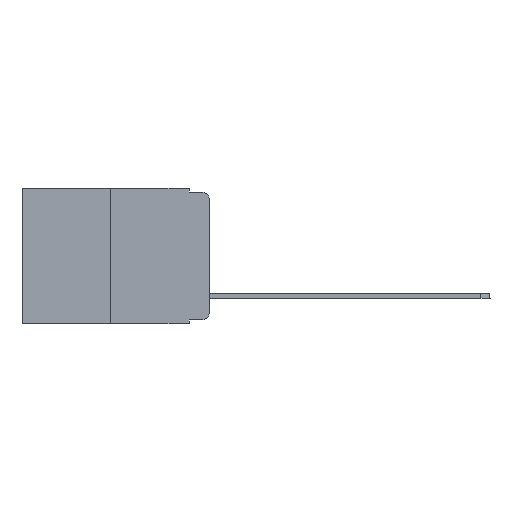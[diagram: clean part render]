
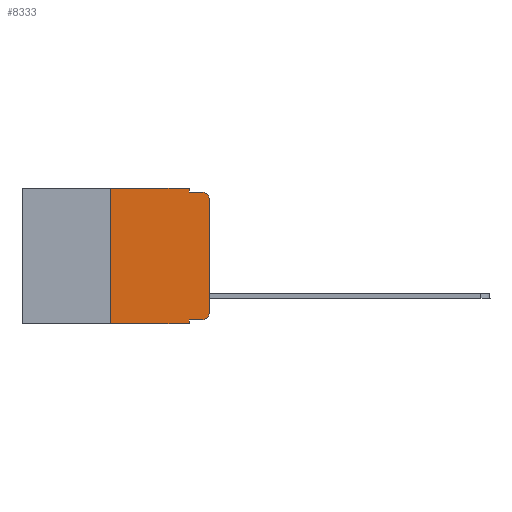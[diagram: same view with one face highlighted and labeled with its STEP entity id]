
A CAD part, left-side view. The second image highlights one B-rep face of the part: STEP entity #8333.
In plain terms, the highlighted planar face has unit normal (-1, 0, 0).
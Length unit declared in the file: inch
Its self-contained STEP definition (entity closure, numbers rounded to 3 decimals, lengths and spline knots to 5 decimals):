
#16 = VERTEX_POINT ( 'NONE', #17097 ) ;
#39 = VECTOR ( 'NONE', #5047, 39.37008 ) ;
#116 = CARTESIAN_POINT ( 'NONE',  ( 0., 0.051, 0. ) ) ;
#132 = EDGE_CURVE ( 'NONE', #12081, #515, #3563, .T. ) ;
#515 = VERTEX_POINT ( 'NONE', #19329 ) ;
#526 = CARTESIAN_POINT ( 'NONE',  ( 0., 0., -0.03 ) ) ;
#568 = EDGE_CURVE ( 'NONE', #9668, #515, #5757, .T. ) ;
#625 = ORIENTED_EDGE ( 'NONE', *, *, #12932, .F. ) ;
#695 = CARTESIAN_POINT ( 'NONE',  ( 0., 0.051, -0.333 ) ) ;
#789 = ORIENTED_EDGE ( 'NONE', *, *, #18024, .T. ) ;
#1224 = CARTESIAN_POINT ( 'NONE',  ( 0., 0.02, -0.333 ) ) ;
#1557 = ORIENTED_EDGE ( 'NONE', *, *, #5802, .T. ) ;
#1624 = ORIENTED_EDGE ( 'NONE', *, *, #2124, .F. ) ;
#1813 = CARTESIAN_POINT ( 'NONE',  ( 0., 0.051, -0.01 ) ) ;
#2092 = ORIENTED_EDGE ( 'NONE', *, *, #11781, .T. ) ;
#2124 = EDGE_CURVE ( 'NONE', #16144, #4587, #16468, .T. ) ;
#2395 = VERTEX_POINT ( 'NONE', #3873 ) ;
#2454 = CARTESIAN_POINT ( 'NONE',  ( 0., 0.473, -0.343 ) ) ;
#2732 = CIRCLE ( 'NONE', #10613, 0.02 ) ;
#2763 = CARTESIAN_POINT ( 'NONE',  ( 0., 0.051, 0. ) ) ;
#2802 = DIRECTION ( 'NONE',  ( -1., 0., 0. ) ) ;
#2873 = DIRECTION ( 'NONE',  ( 1., 0., 0. ) ) ;
#3538 = DIRECTION ( 'NONE',  ( 0., -1., 0. ) ) ;
#3563 = LINE ( 'NONE', #2454, #13452 ) ;
#3873 = CARTESIAN_POINT ( 'NONE',  ( 0., 0., -0.313 ) ) ;
#4555 = CIRCLE ( 'NONE', #14541, 0.02 ) ;
#4587 = VERTEX_POINT ( 'NONE', #8979 ) ;
#4915 = DIRECTION ( 'NONE',  ( 0., 0., 1. ) ) ;
#4970 = DIRECTION ( 'NONE',  ( -1., 0., 0. ) ) ;
#5047 = DIRECTION ( 'NONE',  ( 0., 0., -1. ) ) ;
#5133 = LINE ( 'NONE', #2763, #13836 ) ;
#5757 = LINE ( 'NONE', #116, #39 ) ;
#5802 = EDGE_CURVE ( 'NONE', #2395, #18559, #14811, .T. ) ;
#6745 = VECTOR ( 'NONE', #12735, 39.37008 ) ;
#7552 = VECTOR ( 'NONE', #17179, 39.37008 ) ;
#7692 = PLANE ( 'NONE',  #12149 ) ;
#8035 = LINE ( 'NONE', #18710, #7552 ) ;
#8320 = CARTESIAN_POINT ( 'NONE',  ( 0., 0.25, -0.343 ) ) ;
#8333 = ADVANCED_FACE ( 'NONE', ( #11238 ), #7692, .F. ) ;
#8909 = CARTESIAN_POINT ( 'NONE',  ( 0., 0.051, -0.333 ) ) ;
#8929 = LINE ( 'NONE', #17538, #14399 ) ;
#8979 = CARTESIAN_POINT ( 'NONE',  ( 0., 0.02, -0.01 ) ) ;
#8991 = DIRECTION ( 'NONE',  ( 0., -1., 0. ) ) ;
#9105 = CARTESIAN_POINT ( 'NONE',  ( 0., 0.02, -0.03 ) ) ;
#9374 = CARTESIAN_POINT ( 'NONE',  ( 0., 0.473, 0. ) ) ;
#9668 = VERTEX_POINT ( 'NONE', #8909 ) ;
#10564 = CARTESIAN_POINT ( 'NONE',  ( 0., 0.051, -0.01 ) ) ;
#10613 = AXIS2_PLACEMENT_3D ( 'NONE', #9105, #2802, #13959 ) ;
#10832 = EDGE_CURVE ( 'NONE', #12081, #16, #8929, .T. ) ;
#11146 = DIRECTION ( 'NONE',  ( 0., 0., 1. ) ) ;
#11238 = FACE_OUTER_BOUND ( 'NONE', #15661, .T. ) ;
#11281 = VERTEX_POINT ( 'NONE', #12425 ) ;
#11390 = CARTESIAN_POINT ( 'NONE',  ( 0., 0.02, -0.313 ) ) ;
#11611 = ORIENTED_EDGE ( 'NONE', *, *, #15752, .F. ) ;
#11781 = EDGE_CURVE ( 'NONE', #18559, #4587, #2732, .T. ) ;
#11968 = ORIENTED_EDGE ( 'NONE', *, *, #132, .T. ) ;
#12081 = VERTEX_POINT ( 'NONE', #8320 ) ;
#12149 = AXIS2_PLACEMENT_3D ( 'NONE', #9374, #2873, #17020 ) ;
#12425 = CARTESIAN_POINT ( 'NONE',  ( 0., 0.051, 0. ) ) ;
#12735 = DIRECTION ( 'NONE',  ( 0., -1., 0. ) ) ;
#12932 = EDGE_CURVE ( 'NONE', #11281, #16144, #5133, .T. ) ;
#13411 = VECTOR ( 'NONE', #3538, 39.37008 ) ;
#13452 = VECTOR ( 'NONE', #8991, 39.37008 ) ;
#13836 = VECTOR ( 'NONE', #18351, 39.37008 ) ;
#13959 = DIRECTION ( 'NONE',  ( 0., 0., -1. ) ) ;
#14399 = VECTOR ( 'NONE', #4915, 39.37008 ) ;
#14541 = AXIS2_PLACEMENT_3D ( 'NONE', #11390, #4970, #17666 ) ;
#14811 = LINE ( 'NONE', #15959, #16568 ) ;
#15661 = EDGE_LOOP ( 'NONE', ( #1557, #2092, #1624, #625, #11611, #17527, #11968, #18924, #789, #19433 ) ) ;
#15752 = EDGE_CURVE ( 'NONE', #16, #11281, #8035, .T. ) ;
#15959 = CARTESIAN_POINT ( 'NONE',  ( 0., 0., 0. ) ) ;
#16144 = VERTEX_POINT ( 'NONE', #10564 ) ;
#16468 = LINE ( 'NONE', #1813, #6745 ) ;
#16568 = VECTOR ( 'NONE', #11146, 39.37008 ) ;
#16832 = EDGE_CURVE ( 'NONE', #19651, #2395, #4555, .T. ) ;
#17020 = DIRECTION ( 'NONE',  ( 0., 0., -1. ) ) ;
#17097 = CARTESIAN_POINT ( 'NONE',  ( 0., 0.25, 0. ) ) ;
#17179 = DIRECTION ( 'NONE',  ( 0., -1., 0. ) ) ;
#17527 = ORIENTED_EDGE ( 'NONE', *, *, #10832, .F. ) ;
#17538 = CARTESIAN_POINT ( 'NONE',  ( 0., 0.25, 0. ) ) ;
#17666 = DIRECTION ( 'NONE',  ( 0., 0., -1. ) ) ;
#18024 = EDGE_CURVE ( 'NONE', #9668, #19651, #20112, .T. ) ;
#18351 = DIRECTION ( 'NONE',  ( 0., 0., -1. ) ) ;
#18559 = VERTEX_POINT ( 'NONE', #526 ) ;
#18710 = CARTESIAN_POINT ( 'NONE',  ( 0., 0.473, 0. ) ) ;
#18924 = ORIENTED_EDGE ( 'NONE', *, *, #568, .F. ) ;
#19329 = CARTESIAN_POINT ( 'NONE',  ( 0., 0.051, -0.343 ) ) ;
#19433 = ORIENTED_EDGE ( 'NONE', *, *, #16832, .T. ) ;
#19651 = VERTEX_POINT ( 'NONE', #1224 ) ;
#20112 = LINE ( 'NONE', #695, #13411 ) ;
